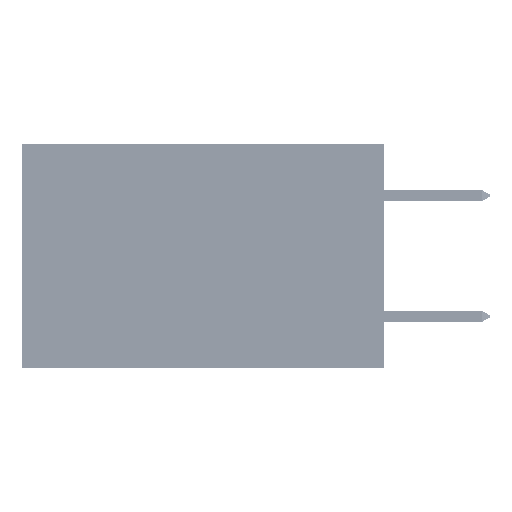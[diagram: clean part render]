
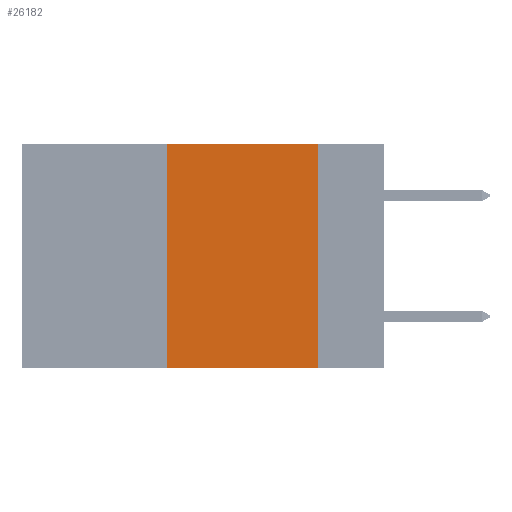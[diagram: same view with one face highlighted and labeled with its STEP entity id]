
A CAD part, left-side view. The second image highlights one B-rep face of the part: STEP entity #26182.
In plain terms, the highlighted planar face has unit normal (-1, 0, 0).
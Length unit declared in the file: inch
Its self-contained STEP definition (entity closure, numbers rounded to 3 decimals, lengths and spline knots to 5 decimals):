
#437 = CARTESIAN_POINT ( 'NONE',  ( 0., 0.11, 0. ) ) ;
#3168 = DIRECTION ( 'NONE',  ( 1., 0., 0. ) ) ;
#5781 = VECTOR ( 'NONE', #7879, 39.37008 ) ;
#6334 = LINE ( 'NONE', #14413, #17185 ) ;
#7098 = ORIENTED_EDGE ( 'NONE', *, *, #14981, .F. ) ;
#7115 = CARTESIAN_POINT ( 'NONE',  ( 0., 0.11, -0.37 ) ) ;
#7879 = DIRECTION ( 'NONE',  ( 0., 0., -1. ) ) ;
#9237 = VERTEX_POINT ( 'NONE', #7115 ) ;
#14165 = CARTESIAN_POINT ( 'NONE',  ( 0., 0.6, 0. ) ) ;
#14413 = CARTESIAN_POINT ( 'NONE',  ( 0., 0.6, -0.37 ) ) ;
#14981 = EDGE_CURVE ( 'NONE', #46216, #29802, #43325, .T. ) ;
#15799 = LINE ( 'NONE', #34387, #34294 ) ;
#17185 = VECTOR ( 'NONE', #18266, 39.37008 ) ;
#18266 = DIRECTION ( 'NONE',  ( 0., -1., 0. ) ) ;
#19966 = CARTESIAN_POINT ( 'NONE',  ( 0., 0.36, 0. ) ) ;
#24821 = DIRECTION ( 'NONE',  ( 0., 0., -1. ) ) ;
#25136 = ORIENTED_EDGE ( 'NONE', *, *, #28930, .T. ) ;
#26182 = ADVANCED_FACE ( 'NONE', ( #45597 ), #31914, .F. ) ;
#27811 = CARTESIAN_POINT ( 'NONE',  ( 0., 0.36, 0. ) ) ;
#28112 = ORIENTED_EDGE ( 'NONE', *, *, #38568, .F. ) ;
#28930 = EDGE_CURVE ( 'NONE', #46216, #9237, #6334, .T. ) ;
#29802 = VERTEX_POINT ( 'NONE', #27811 ) ;
#30138 = ORIENTED_EDGE ( 'NONE', *, *, #40649, .F. ) ;
#30435 = CARTESIAN_POINT ( 'NONE',  ( 0., 0.36, -0.37 ) ) ;
#31447 = AXIS2_PLACEMENT_3D ( 'NONE', #14165, #3168, #24821 ) ;
#31593 = DIRECTION ( 'NONE',  ( 0., 0., 1. ) ) ;
#31914 = PLANE ( 'NONE',  #31447 ) ;
#33320 = CARTESIAN_POINT ( 'NONE',  ( 0., 0.11, 0. ) ) ;
#33952 = EDGE_LOOP ( 'NONE', ( #28112, #30138, #7098, #25136 ) ) ;
#34294 = VECTOR ( 'NONE', #41898, 39.37008 ) ;
#34387 = CARTESIAN_POINT ( 'NONE',  ( 0., 0.6, 0. ) ) ;
#34416 = VERTEX_POINT ( 'NONE', #437 ) ;
#35653 = LINE ( 'NONE', #33320, #5781 ) ;
#38142 = VECTOR ( 'NONE', #31593, 39.37008 ) ;
#38568 = EDGE_CURVE ( 'NONE', #34416, #9237, #35653, .T. ) ;
#40649 = EDGE_CURVE ( 'NONE', #29802, #34416, #15799, .T. ) ;
#41898 = DIRECTION ( 'NONE',  ( 0., -1., 0. ) ) ;
#43325 = LINE ( 'NONE', #19966, #38142 ) ;
#45597 = FACE_OUTER_BOUND ( 'NONE', #33952, .T. ) ;
#46216 = VERTEX_POINT ( 'NONE', #30435 ) ;
